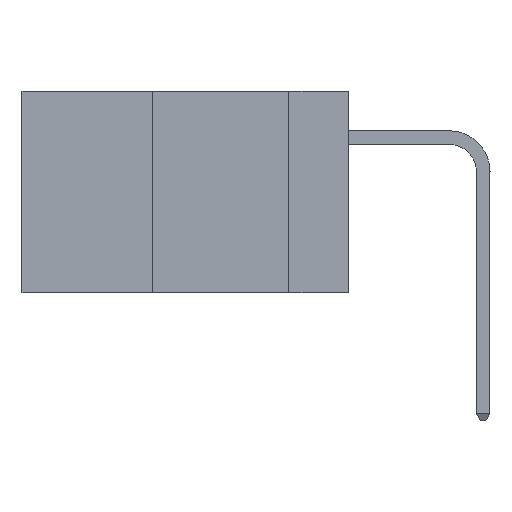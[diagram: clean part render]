
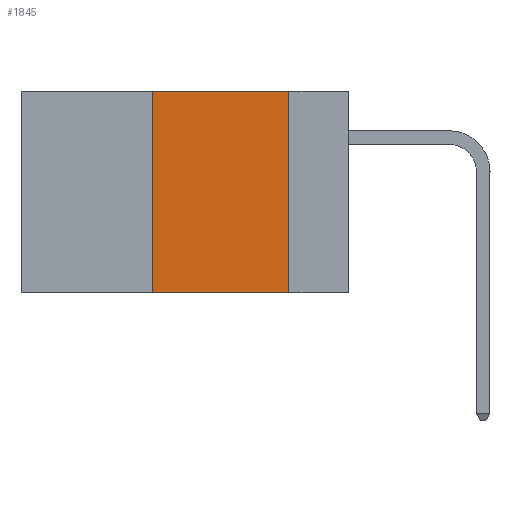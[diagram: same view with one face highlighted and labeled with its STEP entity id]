
A CAD part, left-side view. The second image highlights one B-rep face of the part: STEP entity #1845.
In plain terms, the highlighted planar face has unit normal (-1, 0, 0).
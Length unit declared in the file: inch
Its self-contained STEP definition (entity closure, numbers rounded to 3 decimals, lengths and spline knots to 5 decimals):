
#619 = DIRECTION ( 'NONE',  ( 0., 0., 1. ) ) ;
#1056 = DIRECTION ( 'NONE',  ( 0., 0., -1. ) ) ;
#1140 = DIRECTION ( 'NONE',  ( 1., 0., 0. ) ) ;
#1193 = PLANE ( 'NONE',  #1894 ) ;
#1845 = ADVANCED_FACE ( 'NONE', ( #7917 ), #1193, .F. ) ;
#1894 = AXIS2_PLACEMENT_3D ( 'NONE', #2037, #1140, #1056 ) ;
#2037 = CARTESIAN_POINT ( 'NONE',  ( 0., 0.6, 0. ) ) ;
#2038 = DIRECTION ( 'NONE',  ( 0., -1., 0. ) ) ;
#2140 = LINE ( 'NONE', #13541, #2465 ) ;
#2465 = VECTOR ( 'NONE', #7332, 39.37008 ) ;
#3096 = ORIENTED_EDGE ( 'NONE', *, *, #10114, .F. ) ;
#3130 = VECTOR ( 'NONE', #2038, 39.37008 ) ;
#3145 = ORIENTED_EDGE ( 'NONE', *, *, #5244, .F. ) ;
#3294 = ORIENTED_EDGE ( 'NONE', *, *, #9431, .F. ) ;
#3463 = ORIENTED_EDGE ( 'NONE', *, *, #6546, .T. ) ;
#3800 = EDGE_LOOP ( 'NONE', ( #3096, #3145, #3294, #3463 ) ) ;
#5244 = EDGE_CURVE ( 'NONE', #9744, #10443, #12701, .T. ) ;
#6546 = EDGE_CURVE ( 'NONE', #11673, #13049, #10965, .T. ) ;
#6686 = CARTESIAN_POINT ( 'NONE',  ( 0., 0.36, 0. ) ) ;
#7208 = CARTESIAN_POINT ( 'NONE',  ( 0., 0.36, 0. ) ) ;
#7332 = DIRECTION ( 'NONE',  ( 0., 0., -1. ) ) ;
#7917 = FACE_OUTER_BOUND ( 'NONE', #3800, .T. ) ;
#8861 = CARTESIAN_POINT ( 'NONE',  ( 0., 0.36, -0.37 ) ) ;
#9431 = EDGE_CURVE ( 'NONE', #11673, #9744, #11227, .T. ) ;
#9437 = CARTESIAN_POINT ( 'NONE',  ( 0., 0.6, 0. ) ) ;
#9744 = VERTEX_POINT ( 'NONE', #6686 ) ;
#9979 = VECTOR ( 'NONE', #11495, 39.37008 ) ;
#10114 = EDGE_CURVE ( 'NONE', #10443, #13049, #2140, .T. ) ;
#10279 = CARTESIAN_POINT ( 'NONE',  ( 0., 0.11, -0.37 ) ) ;
#10443 = VERTEX_POINT ( 'NONE', #13038 ) ;
#10965 = LINE ( 'NONE', #13722, #3130 ) ;
#11227 = LINE ( 'NONE', #7208, #12210 ) ;
#11495 = DIRECTION ( 'NONE',  ( 0., -1., 0. ) ) ;
#11673 = VERTEX_POINT ( 'NONE', #8861 ) ;
#12210 = VECTOR ( 'NONE', #619, 39.37008 ) ;
#12701 = LINE ( 'NONE', #9437, #9979 ) ;
#13038 = CARTESIAN_POINT ( 'NONE',  ( 0., 0.11, 0. ) ) ;
#13049 = VERTEX_POINT ( 'NONE', #10279 ) ;
#13541 = CARTESIAN_POINT ( 'NONE',  ( 0., 0.11, 0. ) ) ;
#13722 = CARTESIAN_POINT ( 'NONE',  ( 0., 0.6, -0.37 ) ) ;
